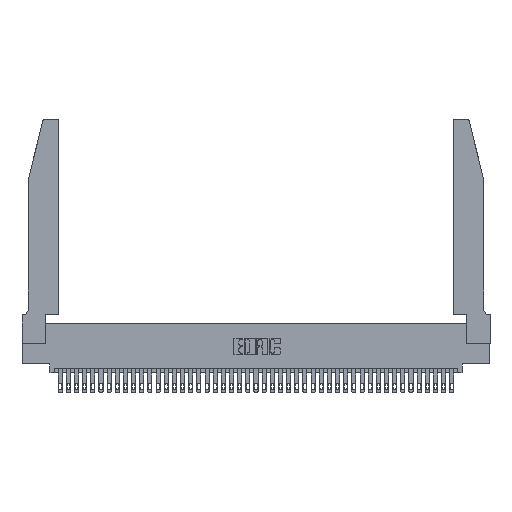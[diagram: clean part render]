
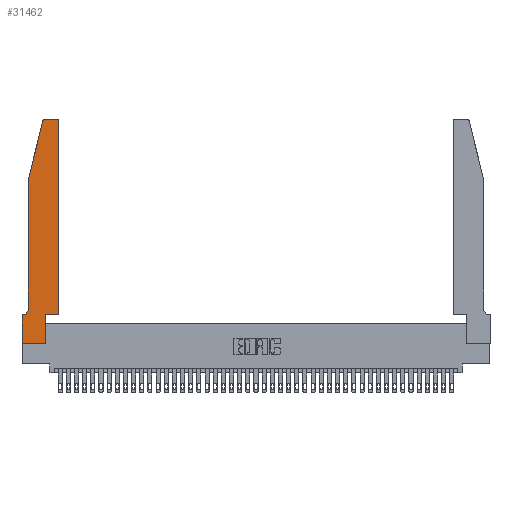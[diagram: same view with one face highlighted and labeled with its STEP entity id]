
A CAD part, top view. The second image highlights one B-rep face of the part: STEP entity #31462.
In plain terms, the highlighted planar face has unit normal (0, 0, 1).
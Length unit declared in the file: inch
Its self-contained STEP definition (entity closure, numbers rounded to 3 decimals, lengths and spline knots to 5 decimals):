
#269 = VECTOR ( 'NONE', #21181, 39.37008 ) ;
#411 = CARTESIAN_POINT ( 'NONE',  ( 0.0755, 0.35, 0.37 ) ) ;
#1760 = LINE ( 'NONE', #7525, #25880 ) ;
#2180 = EDGE_LOOP ( 'NONE', ( #18270, #14578, #21876, #10077, #32687, #19740, #38894, #26889, #32519, #6087, #15611, #9407 ) ) ;
#3058 = VERTEX_POINT ( 'NONE', #29712 ) ;
#3091 = DIRECTION ( 'NONE',  ( -1., 0., 0. ) ) ;
#3116 = AXIS2_PLACEMENT_3D ( 'NONE', #10260, #9720, #27081 ) ;
#3788 = EDGE_CURVE ( 'NONE', #29257, #21134, #31055, .T. ) ;
#4273 = EDGE_CURVE ( 'NONE', #3058, #38202, #38650, .T. ) ;
#4520 = VECTOR ( 'NONE', #41407, 39.37008 ) ;
#5411 = CARTESIAN_POINT ( 'NONE',  ( 0.4505, 2.72, 0.37 ) ) ;
#5520 = VERTEX_POINT ( 'NONE', #17190 ) ;
#5607 = VERTEX_POINT ( 'NONE', #11731 ) ;
#5630 = VECTOR ( 'NONE', #35224, 39.37008 ) ;
#5976 = AXIS2_PLACEMENT_3D ( 'NONE', #29109, #12391, #18932 ) ;
#6087 = ORIENTED_EDGE ( 'NONE', *, *, #24996, .T. ) ;
#6273 = CARTESIAN_POINT ( 'NONE',  ( 0.284, 2.72, 0.37 ) ) ;
#6693 = EDGE_CURVE ( 'NONE', #26540, #37941, #36159, .T. ) ;
#6713 = CARTESIAN_POINT ( 'NONE',  ( 0.2605, 2.75, 0.37 ) ) ;
#6746 = CARTESIAN_POINT ( 'NONE',  ( 0.2865, 0., 0.37 ) ) ;
#7124 = VECTOR ( 'NONE', #25074, 39.37008 ) ;
#7320 = EDGE_CURVE ( 'NONE', #35079, #25504, #35797, .T. ) ;
#7525 = CARTESIAN_POINT ( 'NONE',  ( 0., 0., 0.37 ) ) ;
#9407 = ORIENTED_EDGE ( 'NONE', *, *, #7320, .T. ) ;
#9705 = PLANE ( 'NONE',  #13120 ) ;
#9720 = DIRECTION ( 'NONE',  ( 0., 0., -1. ) ) ;
#10077 = ORIENTED_EDGE ( 'NONE', *, *, #22231, .T. ) ;
#10260 = CARTESIAN_POINT ( 'NONE',  ( 0.0055, 0.42, 0.37 ) ) ;
#10829 = DIRECTION ( 'NONE',  ( 1., 0., 0. ) ) ;
#10850 = CARTESIAN_POINT ( 'NONE',  ( 0.4205, 2.75, 0.37 ) ) ;
#11731 = CARTESIAN_POINT ( 'NONE',  ( 0.0755, 2., 0.37 ) ) ;
#11928 = CARTESIAN_POINT ( 'NONE',  ( 0.2865, 0.35, 0.37 ) ) ;
#12391 = DIRECTION ( 'NONE',  ( 0., 0., 1. ) ) ;
#13120 = AXIS2_PLACEMENT_3D ( 'NONE', #33528, #19678, #36764 ) ;
#14578 = ORIENTED_EDGE ( 'NONE', *, *, #6693, .T. ) ;
#15611 = ORIENTED_EDGE ( 'NONE', *, *, #28884, .T. ) ;
#16303 = EDGE_CURVE ( 'NONE', #24091, #5520, #18352, .T. ) ;
#16806 = CARTESIAN_POINT ( 'NONE',  ( 0.4505, 0.35, 0.37 ) ) ;
#16970 = CARTESIAN_POINT ( 'NONE',  ( 0.284, 2.75, 0.37 ) ) ;
#17190 = CARTESIAN_POINT ( 'NONE',  ( 0.2865, 0.35, 0.37 ) ) ;
#17578 = DIRECTION ( 'NONE',  ( -1., 0., 0. ) ) ;
#18129 = EDGE_CURVE ( 'NONE', #21134, #3058, #27828, .T. ) ;
#18270 = ORIENTED_EDGE ( 'NONE', *, *, #22352, .T. ) ;
#18352 = LINE ( 'NONE', #11928, #7124 ) ;
#18932 = DIRECTION ( 'NONE',  ( 1., 0., 0. ) ) ;
#19678 = DIRECTION ( 'NONE',  ( 0., 0., 1. ) ) ;
#19740 = ORIENTED_EDGE ( 'NONE', *, *, #18129, .T. ) ;
#20960 = LINE ( 'NONE', #38360, #5630 ) ;
#21134 = VERTEX_POINT ( 'NONE', #24504 ) ;
#21181 = DIRECTION ( 'NONE',  ( 1., 0., 0. ) ) ;
#21683 = VECTOR ( 'NONE', #17578, 39.37008 ) ;
#21876 = ORIENTED_EDGE ( 'NONE', *, *, #40821, .T. ) ;
#22231 = EDGE_CURVE ( 'NONE', #5607, #29257, #24036, .T. ) ;
#22352 = EDGE_CURVE ( 'NONE', #25504, #26540, #36763, .T. ) ;
#23200 = CARTESIAN_POINT ( 'NONE',  ( 0., 0., 0.37 ) ) ;
#24036 = LINE ( 'NONE', #38418, #4520 ) ;
#24091 = VERTEX_POINT ( 'NONE', #6746 ) ;
#24504 = CARTESIAN_POINT ( 'NONE',  ( 0.0055, 0.35, 0.37 ) ) ;
#24996 = EDGE_CURVE ( 'NONE', #5520, #25466, #36142, .T. ) ;
#25074 = DIRECTION ( 'NONE',  ( 0., 1., 0. ) ) ;
#25093 = CARTESIAN_POINT ( 'NONE',  ( 0.25487, 2.72718, 0.37 ) ) ;
#25466 = VERTEX_POINT ( 'NONE', #16806 ) ;
#25504 = VERTEX_POINT ( 'NONE', #10850 ) ;
#25706 = DIRECTION ( 'NONE',  ( 0., 0., 1. ) ) ;
#25880 = VECTOR ( 'NONE', #10829, 39.37008 ) ;
#26540 = VERTEX_POINT ( 'NONE', #16970 ) ;
#26889 = ORIENTED_EDGE ( 'NONE', *, *, #31493, .T. ) ;
#27041 = CARTESIAN_POINT ( 'NONE',  ( 0.0755, 0.42, 0.37 ) ) ;
#27080 = VECTOR ( 'NONE', #3091, 39.37008 ) ;
#27081 = DIRECTION ( 'NONE',  ( -1., 0., 0. ) ) ;
#27828 = LINE ( 'NONE', #411, #21683 ) ;
#28884 = EDGE_CURVE ( 'NONE', #25466, #35079, #20960, .T. ) ;
#29109 = CARTESIAN_POINT ( 'NONE',  ( 0.4205, 2.72, 0.37 ) ) ;
#29257 = VERTEX_POINT ( 'NONE', #27041 ) ;
#29712 = CARTESIAN_POINT ( 'NONE',  ( 0., 0.35, 0.37 ) ) ;
#29971 = VECTOR ( 'NONE', #30756, 39.37008 ) ;
#30756 = DIRECTION ( 'NONE',  ( 0., -1., 0. ) ) ;
#31055 = CIRCLE ( 'NONE', #3116, 0.07 ) ;
#31232 = DIRECTION ( 'NONE',  ( -0.239, -0.971, 0. ) ) ;
#31462 = ADVANCED_FACE ( 'NONE', ( #41162 ), #9705, .T. ) ;
#31493 = EDGE_CURVE ( 'NONE', #38202, #24091, #1760, .T. ) ;
#31647 = CARTESIAN_POINT ( 'NONE',  ( 0.0755, 2., 0.37 ) ) ;
#31703 = AXIS2_PLACEMENT_3D ( 'NONE', #6273, #25706, #38957 ) ;
#32519 = ORIENTED_EDGE ( 'NONE', *, *, #16303, .T. ) ;
#32687 = ORIENTED_EDGE ( 'NONE', *, *, #3788, .T. ) ;
#33528 = CARTESIAN_POINT ( 'NONE',  ( 0., 0.35, 0.37 ) ) ;
#33875 = CARTESIAN_POINT ( 'NONE',  ( 0., 0., 0.37 ) ) ;
#35079 = VERTEX_POINT ( 'NONE', #5411 ) ;
#35224 = DIRECTION ( 'NONE',  ( 0., 1., 0. ) ) ;
#35797 = CIRCLE ( 'NONE', #5976, 0.03 ) ;
#36142 = LINE ( 'NONE', #37582, #269 ) ;
#36159 = CIRCLE ( 'NONE', #31703, 0.03 ) ;
#36763 = LINE ( 'NONE', #6713, #27080 ) ;
#36764 = DIRECTION ( 'NONE',  ( 1., 0., 0. ) ) ;
#36871 = VECTOR ( 'NONE', #31232, 39.37008 ) ;
#37582 = CARTESIAN_POINT ( 'NONE',  ( 0.4505, 0.35, 0.37 ) ) ;
#37941 = VERTEX_POINT ( 'NONE', #25093 ) ;
#38202 = VERTEX_POINT ( 'NONE', #23200 ) ;
#38360 = CARTESIAN_POINT ( 'NONE',  ( 0.4505, 0.35, 0.37 ) ) ;
#38418 = CARTESIAN_POINT ( 'NONE',  ( 0.0755, 2., 0.37 ) ) ;
#38650 = LINE ( 'NONE', #33875, #29971 ) ;
#38894 = ORIENTED_EDGE ( 'NONE', *, *, #4273, .T. ) ;
#38957 = DIRECTION ( 'NONE',  ( 1., 0., 0. ) ) ;
#40473 = LINE ( 'NONE', #31647, #36871 ) ;
#40821 = EDGE_CURVE ( 'NONE', #37941, #5607, #40473, .T. ) ;
#41162 = FACE_OUTER_BOUND ( 'NONE', #2180, .T. ) ;
#41407 = DIRECTION ( 'NONE',  ( 0., -1., 0. ) ) ;
